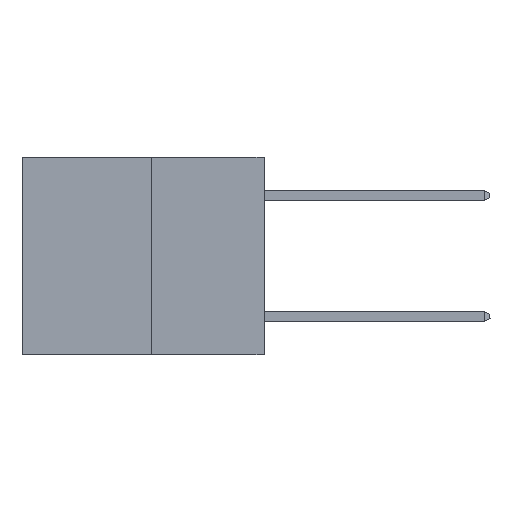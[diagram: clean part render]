
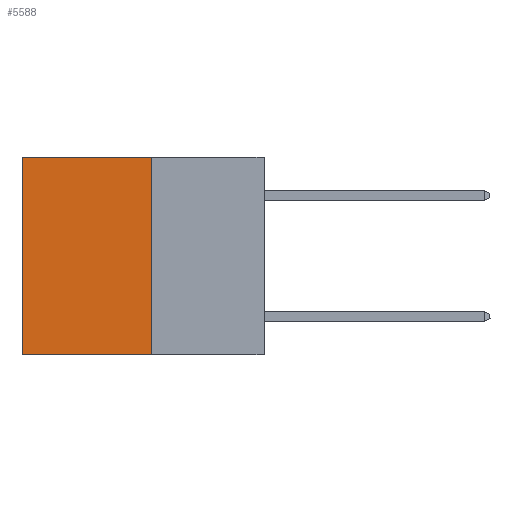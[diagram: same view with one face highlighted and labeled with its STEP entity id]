
A CAD part, left-side view. The second image highlights one B-rep face of the part: STEP entity #5588.
In plain terms, the highlighted planar face has unit normal (-1, 0, 0).
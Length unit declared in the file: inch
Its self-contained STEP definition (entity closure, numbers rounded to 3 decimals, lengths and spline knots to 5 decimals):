
#601 = LINE ( 'NONE', #15109, #17278 ) ;
#705 = CARTESIAN_POINT ( 'NONE',  ( 0.3165, 0.6, -0.49 ) ) ;
#3521 = DIRECTION ( 'NONE',  ( 0., 1., 0. ) ) ;
#3975 = VERTEX_POINT ( 'NONE', #705 ) ;
#4227 = DIRECTION ( 'NONE',  ( 1., 0., 0. ) ) ;
#4580 = ORIENTED_EDGE ( 'NONE', *, *, #10853, .F. ) ;
#5120 = ORIENTED_EDGE ( 'NONE', *, *, #14293, .F. ) ;
#5588 = ADVANCED_FACE ( 'NONE', ( #19700 ), #10608, .F. ) ;
#6441 = ORIENTED_EDGE ( 'NONE', *, *, #18212, .T. ) ;
#6672 = ORIENTED_EDGE ( 'NONE', *, *, #10826, .T. ) ;
#6881 = LINE ( 'NONE', #11834, #10180 ) ;
#9091 = VERTEX_POINT ( 'NONE', #13057 ) ;
#9232 = DIRECTION ( 'NONE',  ( 0., 0., -1. ) ) ;
#9384 = VERTEX_POINT ( 'NONE', #12066 ) ;
#10180 = VECTOR ( 'NONE', #19830, 39.37008 ) ;
#10425 = VERTEX_POINT ( 'NONE', #17716 ) ;
#10608 = PLANE ( 'NONE',  #19970 ) ;
#10826 = EDGE_CURVE ( 'NONE', #10425, #3975, #6881, .T. ) ;
#10853 = EDGE_CURVE ( 'NONE', #9384, #9091, #601, .T. ) ;
#11192 = CARTESIAN_POINT ( 'NONE',  ( 0.3165, 0.28, -0.49 ) ) ;
#11834 = CARTESIAN_POINT ( 'NONE',  ( 0.3165, 0.6, -0.49 ) ) ;
#12066 = CARTESIAN_POINT ( 'NONE',  ( 0.3165, 0.28, 0. ) ) ;
#12284 = CARTESIAN_POINT ( 'NONE',  ( 0.3165, 0.28, -0.49 ) ) ;
#12617 = EDGE_LOOP ( 'NONE', ( #6672, #5120, #4580, #6441 ) ) ;
#13057 = CARTESIAN_POINT ( 'NONE',  ( 0.3165, 0.28, -0.49 ) ) ;
#13088 = DIRECTION ( 'NONE',  ( 0., 1., 0. ) ) ;
#13403 = DIRECTION ( 'NONE',  ( 0., 0., -1. ) ) ;
#14293 = EDGE_CURVE ( 'NONE', #9091, #3975, #15303, .T. ) ;
#15109 = CARTESIAN_POINT ( 'NONE',  ( 0.3165, 0.28, -0.49 ) ) ;
#15303 = LINE ( 'NONE', #11192, #15809 ) ;
#15354 = LINE ( 'NONE', #18105, #17664 ) ;
#15809 = VECTOR ( 'NONE', #13088, 39.37008 ) ;
#17278 = VECTOR ( 'NONE', #13403, 39.37008 ) ;
#17664 = VECTOR ( 'NONE', #3521, 39.37008 ) ;
#17716 = CARTESIAN_POINT ( 'NONE',  ( 0.3165, 0.6, 0. ) ) ;
#18105 = CARTESIAN_POINT ( 'NONE',  ( 0.3165, 0.28, 0. ) ) ;
#18212 = EDGE_CURVE ( 'NONE', #9384, #10425, #15354, .T. ) ;
#19700 = FACE_OUTER_BOUND ( 'NONE', #12617, .T. ) ;
#19830 = DIRECTION ( 'NONE',  ( 0., 0., -1. ) ) ;
#19970 = AXIS2_PLACEMENT_3D ( 'NONE', #12284, #4227, #9232 ) ;
